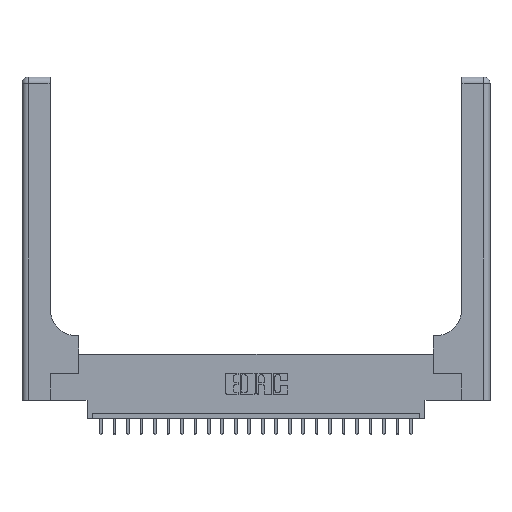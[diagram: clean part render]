
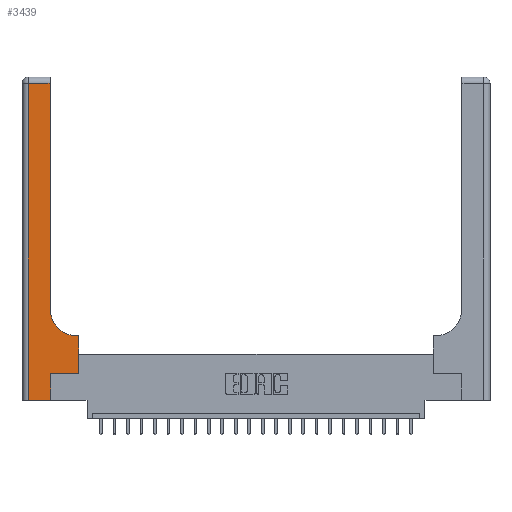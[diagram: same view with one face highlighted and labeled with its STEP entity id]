
A CAD part, top view. The second image highlights one B-rep face of the part: STEP entity #3439.
In plain terms, the highlighted planar face has unit normal (0, 0, 1).
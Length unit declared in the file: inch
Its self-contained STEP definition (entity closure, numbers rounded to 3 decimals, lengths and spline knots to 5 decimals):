
#112 = EDGE_CURVE ( 'NONE', #17030, #600, #16671, .T. ) ;
#301 = EDGE_CURVE ( 'NONE', #2511, #22965, #14808, .T. ) ;
#600 = VERTEX_POINT ( 'NONE', #14588 ) ;
#715 = DIRECTION ( 'NONE',  ( 0., -1., 0. ) ) ;
#861 = CARTESIAN_POINT ( 'NONE',  ( 0.26, 2.94, 0.37 ) ) ;
#1303 = LINE ( 'NONE', #15390, #10802 ) ;
#1375 = CARTESIAN_POINT ( 'NONE',  ( 0.51, 0.85, 0.37 ) ) ;
#1737 = CARTESIAN_POINT ( 'NONE',  ( 0.528, 0.25, 0.37 ) ) ;
#1971 = EDGE_CURVE ( 'NONE', #22965, #4331, #13776, .T. ) ;
#2506 = VERTEX_POINT ( 'NONE', #9383 ) ;
#2511 = VERTEX_POINT ( 'NONE', #19774 ) ;
#2655 = VERTEX_POINT ( 'NONE', #861 ) ;
#2903 = LINE ( 'NONE', #10046, #10958 ) ;
#3125 = AXIS2_PLACEMENT_3D ( 'NONE', #19608, #21588, #12702 ) ;
#3439 = ADVANCED_FACE ( 'NONE', ( #15955 ), #9333, .F. ) ;
#3847 = VECTOR ( 'NONE', #10956, 39.37008 ) ;
#4331 = VERTEX_POINT ( 'NONE', #10567 ) ;
#4407 = EDGE_CURVE ( 'NONE', #2655, #17030, #2903, .T. ) ;
#4767 = ORIENTED_EDGE ( 'NONE', *, *, #4407, .T. ) ;
#4856 = VECTOR ( 'NONE', #7176, 39.37008 ) ;
#5133 = ORIENTED_EDGE ( 'NONE', *, *, #21245, .T. ) ;
#5550 = ORIENTED_EDGE ( 'NONE', *, *, #15109, .T. ) ;
#7176 = DIRECTION ( 'NONE',  ( 0., 1., 0. ) ) ;
#7568 = EDGE_CURVE ( 'NONE', #4331, #17162, #15770, .T. ) ;
#7599 = EDGE_LOOP ( 'NONE', ( #5550, #4767, #13728, #21503, #5133, #13122, #20810, #22325, #21678 ) ) ;
#8523 = VECTOR ( 'NONE', #15538, 39.37008 ) ;
#9259 = EDGE_CURVE ( 'NONE', #600, #23059, #15847, .T. ) ;
#9333 = PLANE ( 'NONE',  #3125 ) ;
#9383 = CARTESIAN_POINT ( 'NONE',  ( 0.26, 0.85, 0.37 ) ) ;
#10046 = CARTESIAN_POINT ( 'NONE',  ( 0., 2.94, 0.37 ) ) ;
#10567 = CARTESIAN_POINT ( 'NONE',  ( 0.528, 0.6, 0.37 ) ) ;
#10802 = VECTOR ( 'NONE', #22544, 39.37008 ) ;
#10866 = VECTOR ( 'NONE', #13060, 39.37008 ) ;
#10956 = DIRECTION ( 'NONE',  ( 0., 1., 0. ) ) ;
#10958 = VECTOR ( 'NONE', #20695, 39.37008 ) ;
#11125 = VECTOR ( 'NONE', #715, 39.37008 ) ;
#11667 = CARTESIAN_POINT ( 'NONE',  ( 0.06, 3., 0.37 ) ) ;
#11860 = DIRECTION ( 'NONE',  ( 0., 0., -1. ) ) ;
#12702 = DIRECTION ( 'NONE',  ( -1., 0., 0. ) ) ;
#13060 = DIRECTION ( 'NONE',  ( 1., 0., 0. ) ) ;
#13122 = ORIENTED_EDGE ( 'NONE', *, *, #301, .T. ) ;
#13728 = ORIENTED_EDGE ( 'NONE', *, *, #112, .T. ) ;
#13776 = LINE ( 'NONE', #1737, #3847 ) ;
#14135 = DIRECTION ( 'NONE',  ( 1., 0., 0. ) ) ;
#14333 = CARTESIAN_POINT ( 'NONE',  ( 0.528, 0.25, 0.37 ) ) ;
#14458 = EDGE_CURVE ( 'NONE', #17162, #2506, #18247, .T. ) ;
#14588 = CARTESIAN_POINT ( 'NONE',  ( 0.06, 0., 0.37 ) ) ;
#14808 = LINE ( 'NONE', #21954, #10866 ) ;
#15109 = EDGE_CURVE ( 'NONE', #2506, #2655, #17775, .T. ) ;
#15242 = AXIS2_PLACEMENT_3D ( 'NONE', #1375, #11860, #19109 ) ;
#15390 = CARTESIAN_POINT ( 'NONE',  ( 0.265, 0., 0.37 ) ) ;
#15538 = DIRECTION ( 'NONE',  ( -1., 0., 0. ) ) ;
#15770 = LINE ( 'NONE', #22583, #8523 ) ;
#15797 = CARTESIAN_POINT ( 'NONE',  ( 0.06, 2.94, 0.37 ) ) ;
#15847 = LINE ( 'NONE', #19144, #19571 ) ;
#15955 = FACE_OUTER_BOUND ( 'NONE', #7599, .T. ) ;
#16022 = CARTESIAN_POINT ( 'NONE',  ( 0.26, 3., 0.37 ) ) ;
#16671 = LINE ( 'NONE', #11667, #11125 ) ;
#17030 = VERTEX_POINT ( 'NONE', #15797 ) ;
#17162 = VERTEX_POINT ( 'NONE', #18489 ) ;
#17775 = LINE ( 'NONE', #16022, #4856 ) ;
#17929 = CARTESIAN_POINT ( 'NONE',  ( 0.265, 0., 0.37 ) ) ;
#18247 = CIRCLE ( 'NONE', #15242, 0.25 ) ;
#18489 = CARTESIAN_POINT ( 'NONE',  ( 0.51, 0.6, 0.37 ) ) ;
#19109 = DIRECTION ( 'NONE',  ( 1., 0., 0. ) ) ;
#19144 = CARTESIAN_POINT ( 'NONE',  ( 0., 0., 0.37 ) ) ;
#19571 = VECTOR ( 'NONE', #14135, 39.37008 ) ;
#19608 = CARTESIAN_POINT ( 'NONE',  ( 0., 3., 0.37 ) ) ;
#19774 = CARTESIAN_POINT ( 'NONE',  ( 0.265, 0.25, 0.37 ) ) ;
#20695 = DIRECTION ( 'NONE',  ( -1., 0., 0. ) ) ;
#20810 = ORIENTED_EDGE ( 'NONE', *, *, #1971, .T. ) ;
#21245 = EDGE_CURVE ( 'NONE', #23059, #2511, #1303, .T. ) ;
#21503 = ORIENTED_EDGE ( 'NONE', *, *, #9259, .T. ) ;
#21588 = DIRECTION ( 'NONE',  ( 0., 0., -1. ) ) ;
#21678 = ORIENTED_EDGE ( 'NONE', *, *, #14458, .T. ) ;
#21954 = CARTESIAN_POINT ( 'NONE',  ( 0.265, 0.25, 0.37 ) ) ;
#22325 = ORIENTED_EDGE ( 'NONE', *, *, #7568, .T. ) ;
#22544 = DIRECTION ( 'NONE',  ( 0., 1., 0. ) ) ;
#22583 = CARTESIAN_POINT ( 'NONE',  ( 0.26, 0.6, 0.37 ) ) ;
#22965 = VERTEX_POINT ( 'NONE', #14333 ) ;
#23059 = VERTEX_POINT ( 'NONE', #17929 ) ;
